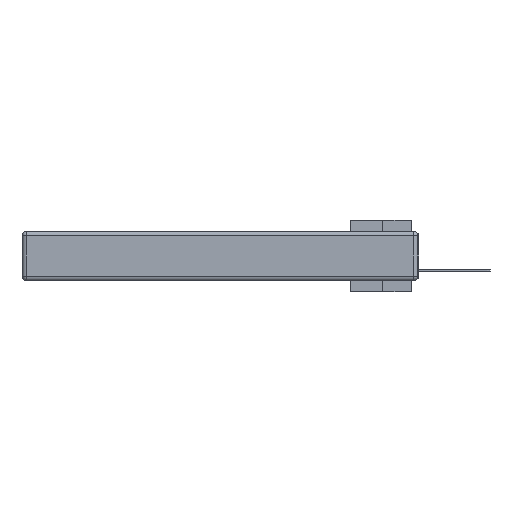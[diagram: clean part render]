
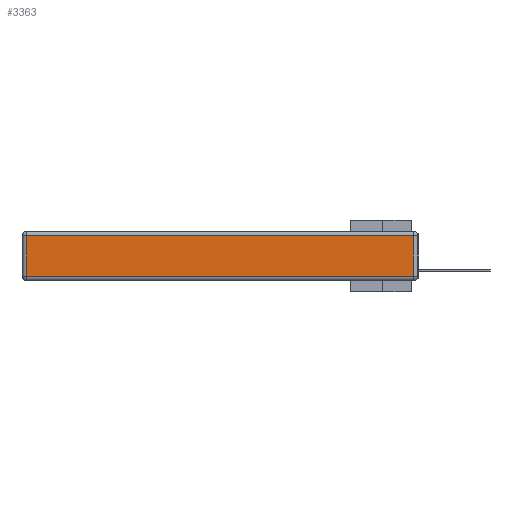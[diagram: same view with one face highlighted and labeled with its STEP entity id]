
A CAD part, left-side view. The second image highlights one B-rep face of the part: STEP entity #3363.
In plain terms, the highlighted planar face has unit normal (-1, 0, 0).
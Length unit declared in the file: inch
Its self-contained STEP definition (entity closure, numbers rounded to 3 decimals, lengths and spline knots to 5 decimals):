
#1681 = CARTESIAN_POINT ( 'NONE',  ( 0., 2.72, -0.313 ) ) ;
#2412 = ORIENTED_EDGE ( 'NONE', *, *, #18308, .T. ) ;
#3363 = ADVANCED_FACE ( 'NONE', ( #37593 ), #9127, .T. ) ;
#3495 = ORIENTED_EDGE ( 'NONE', *, *, #7716, .T. ) ;
#5320 = VECTOR ( 'NONE', #31290, 39.37008 ) ;
#6791 = LINE ( 'NONE', #25763, #37459 ) ;
#7716 = EDGE_CURVE ( 'NONE', #20534, #13437, #12203, .T. ) ;
#8473 = CARTESIAN_POINT ( 'NONE',  ( 0., 2.72, -0.03 ) ) ;
#8987 = DIRECTION ( 'NONE',  ( -1., 0., 0. ) ) ;
#9127 = PLANE ( 'NONE',  #11921 ) ;
#9536 = DIRECTION ( 'NONE',  ( 0., 0., -1. ) ) ;
#9783 = LINE ( 'NONE', #24790, #5320 ) ;
#11921 = AXIS2_PLACEMENT_3D ( 'NONE', #31005, #8987, #27825 ) ;
#12203 = LINE ( 'NONE', #40795, #18630 ) ;
#13437 = VERTEX_POINT ( 'NONE', #1681 ) ;
#14697 = CARTESIAN_POINT ( 'NONE',  ( 0., 0.03, -0.313 ) ) ;
#15706 = VECTOR ( 'NONE', #24358, 39.37008 ) ;
#16071 = VERTEX_POINT ( 'NONE', #14697 ) ;
#16848 = ORIENTED_EDGE ( 'NONE', *, *, #37174, .T. ) ;
#18038 = CARTESIAN_POINT ( 'NONE',  ( 0., 0., -0.313 ) ) ;
#18308 = EDGE_CURVE ( 'NONE', #16071, #19693, #9783, .T. ) ;
#18630 = VECTOR ( 'NONE', #9536, 39.37008 ) ;
#19253 = ORIENTED_EDGE ( 'NONE', *, *, #27932, .T. ) ;
#19693 = VERTEX_POINT ( 'NONE', #26275 ) ;
#20534 = VERTEX_POINT ( 'NONE', #8473 ) ;
#21501 = EDGE_LOOP ( 'NONE', ( #19253, #2412, #16848, #3495 ) ) ;
#24358 = DIRECTION ( 'NONE',  ( 0., -1., 0. ) ) ;
#24790 = CARTESIAN_POINT ( 'NONE',  ( 0., 0.03, -0.343 ) ) ;
#25064 = LINE ( 'NONE', #18038, #15706 ) ;
#25763 = CARTESIAN_POINT ( 'NONE',  ( 0., 2.75, -0.03 ) ) ;
#26275 = CARTESIAN_POINT ( 'NONE',  ( 0., 0.03, -0.03 ) ) ;
#27825 = DIRECTION ( 'NONE',  ( 0., 0., 1. ) ) ;
#27932 = EDGE_CURVE ( 'NONE', #13437, #16071, #25064, .T. ) ;
#31005 = CARTESIAN_POINT ( 'NONE',  ( 0., 0., -0.343 ) ) ;
#31290 = DIRECTION ( 'NONE',  ( 0., 0., 1. ) ) ;
#37174 = EDGE_CURVE ( 'NONE', #19693, #20534, #6791, .T. ) ;
#37459 = VECTOR ( 'NONE', #37932, 39.37008 ) ;
#37593 = FACE_OUTER_BOUND ( 'NONE', #21501, .T. ) ;
#37932 = DIRECTION ( 'NONE',  ( 0., 1., 0. ) ) ;
#40795 = CARTESIAN_POINT ( 'NONE',  ( 0., 2.72, -0.343 ) ) ;
